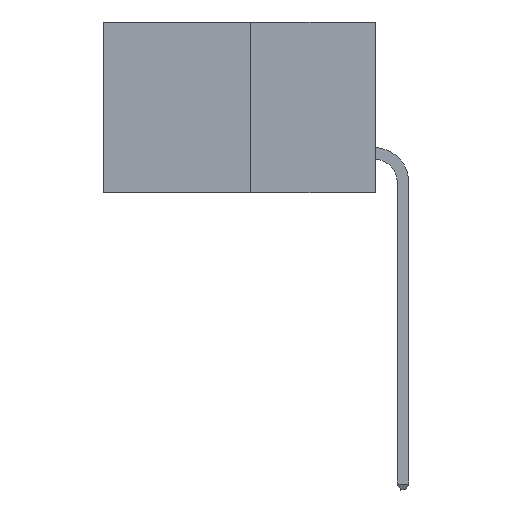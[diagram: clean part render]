
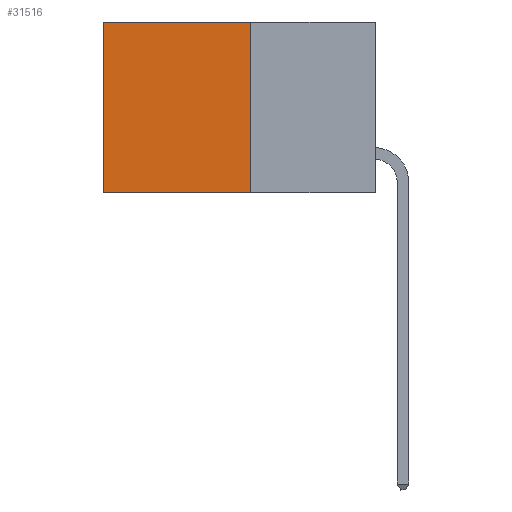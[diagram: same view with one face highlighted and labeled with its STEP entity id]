
A CAD part, left-side view. The second image highlights one B-rep face of the part: STEP entity #31516.
In plain terms, the highlighted planar face has unit normal (-1, 0, 0).
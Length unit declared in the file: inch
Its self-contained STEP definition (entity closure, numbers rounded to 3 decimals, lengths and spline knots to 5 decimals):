
#541 = EDGE_CURVE ( 'NONE', #17797, #21305, #9765, .T. ) ;
#2004 = FACE_OUTER_BOUND ( 'NONE', #2644, .T. ) ;
#2418 = ORIENTED_EDGE ( 'NONE', *, *, #8941, .F. ) ;
#2644 = EDGE_LOOP ( 'NONE', ( #3168, #31052, #2418, #10799 ) ) ;
#3168 = ORIENTED_EDGE ( 'NONE', *, *, #20464, .T. ) ;
#4249 = VERTEX_POINT ( 'NONE', #26984 ) ;
#4545 = DIRECTION ( 'NONE',  ( 0., 0., -1. ) ) ;
#5023 = AXIS2_PLACEMENT_3D ( 'NONE', #26000, #31036, #16108 ) ;
#7580 = LINE ( 'NONE', #22978, #27005 ) ;
#8941 = EDGE_CURVE ( 'NONE', #17797, #4249, #7580, .T. ) ;
#8942 = VECTOR ( 'NONE', #14159, 39.37008 ) ;
#9170 = CARTESIAN_POINT ( 'NONE',  ( 0.277, 0.27, 0. ) ) ;
#9765 = LINE ( 'NONE', #16592, #8942 ) ;
#10799 = ORIENTED_EDGE ( 'NONE', *, *, #541, .T. ) ;
#10977 = DIRECTION ( 'NONE',  ( 0., 0., -1. ) ) ;
#12490 = CARTESIAN_POINT ( 'NONE',  ( 0.277, 0.59, -0.37 ) ) ;
#13522 = LINE ( 'NONE', #12490, #32709 ) ;
#14159 = DIRECTION ( 'NONE',  ( 0., 1., 0. ) ) ;
#16108 = DIRECTION ( 'NONE',  ( 0., 0., -1. ) ) ;
#16592 = CARTESIAN_POINT ( 'NONE',  ( 0.277, 0.27, 0. ) ) ;
#17797 = VERTEX_POINT ( 'NONE', #9170 ) ;
#18333 = VECTOR ( 'NONE', #30196, 39.37008 ) ;
#20155 = CARTESIAN_POINT ( 'NONE',  ( 0.277, 0.27, -0.37 ) ) ;
#20464 = EDGE_CURVE ( 'NONE', #21305, #20574, #13522, .T. ) ;
#20574 = VERTEX_POINT ( 'NONE', #32877 ) ;
#20984 = PLANE ( 'NONE',  #5023 ) ;
#21305 = VERTEX_POINT ( 'NONE', #22961 ) ;
#22961 = CARTESIAN_POINT ( 'NONE',  ( 0.277, 0.59, 0. ) ) ;
#22978 = CARTESIAN_POINT ( 'NONE',  ( 0.277, 0.27, -0.37 ) ) ;
#24952 = LINE ( 'NONE', #20155, #18333 ) ;
#26000 = CARTESIAN_POINT ( 'NONE',  ( 0.277, 0.27, -0.37 ) ) ;
#26984 = CARTESIAN_POINT ( 'NONE',  ( 0.277, 0.27, -0.37 ) ) ;
#27005 = VECTOR ( 'NONE', #10977, 39.37008 ) ;
#30196 = DIRECTION ( 'NONE',  ( 0., 1., 0. ) ) ;
#30576 = EDGE_CURVE ( 'NONE', #4249, #20574, #24952, .T. ) ;
#31036 = DIRECTION ( 'NONE',  ( 1., 0., 0. ) ) ;
#31052 = ORIENTED_EDGE ( 'NONE', *, *, #30576, .F. ) ;
#31516 = ADVANCED_FACE ( 'NONE', ( #2004 ), #20984, .F. ) ;
#32709 = VECTOR ( 'NONE', #4545, 39.37008 ) ;
#32877 = CARTESIAN_POINT ( 'NONE',  ( 0.277, 0.59, -0.37 ) ) ;
